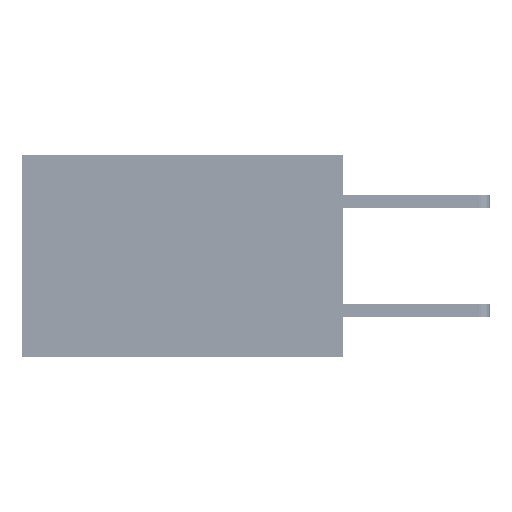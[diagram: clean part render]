
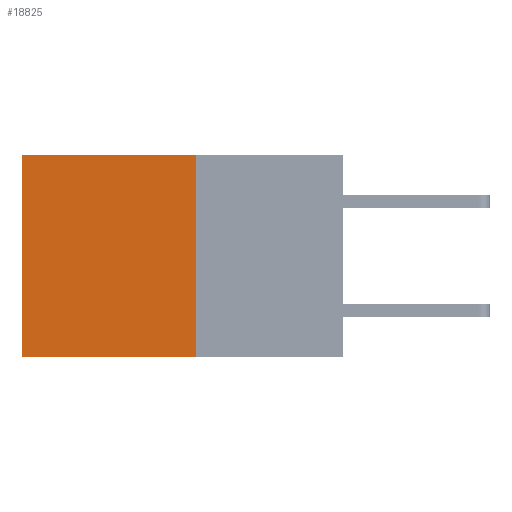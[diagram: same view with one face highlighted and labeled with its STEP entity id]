
A CAD part, left-side view. The second image highlights one B-rep face of the part: STEP entity #18825.
In plain terms, the highlighted planar face has unit normal (-1, 0, 0).
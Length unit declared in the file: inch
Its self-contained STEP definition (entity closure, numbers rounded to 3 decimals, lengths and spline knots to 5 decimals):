
#431 = FACE_OUTER_BOUND ( 'NONE', #22893, .T. ) ;
#1126 = CARTESIAN_POINT ( 'NONE',  ( 0.277, 0.27, 0. ) ) ;
#1893 = ORIENTED_EDGE ( 'NONE', *, *, #12973, .T. ) ;
#2403 = LINE ( 'NONE', #24866, #23224 ) ;
#3256 = CARTESIAN_POINT ( 'NONE',  ( 0.277, 0.59, 0. ) ) ;
#5105 = VERTEX_POINT ( 'NONE', #3256 ) ;
#5894 = DIRECTION ( 'NONE',  ( 1., 0., 0. ) ) ;
#6621 = CARTESIAN_POINT ( 'NONE',  ( 0.277, 0.27, -0.37 ) ) ;
#6742 = VECTOR ( 'NONE', #28355, 39.37008 ) ;
#7598 = ORIENTED_EDGE ( 'NONE', *, *, #15691, .T. ) ;
#7933 = VECTOR ( 'NONE', #16899, 39.37008 ) ;
#10224 = AXIS2_PLACEMENT_3D ( 'NONE', #14070, #5894, #19494 ) ;
#12973 = EDGE_CURVE ( 'NONE', #5105, #17827, #33513, .T. ) ;
#13945 = DIRECTION ( 'NONE',  ( 0., 0., -1. ) ) ;
#14070 = CARTESIAN_POINT ( 'NONE',  ( 0.277, 0.27, -0.37 ) ) ;
#14175 = CARTESIAN_POINT ( 'NONE',  ( 0.277, 0.27, 0. ) ) ;
#15649 = EDGE_CURVE ( 'NONE', #16264, #22211, #2403, .T. ) ;
#15691 = EDGE_CURVE ( 'NONE', #16264, #5105, #30457, .T. ) ;
#16264 = VERTEX_POINT ( 'NONE', #1126 ) ;
#16786 = PLANE ( 'NONE',  #10224 ) ;
#16899 = DIRECTION ( 'NONE',  ( 0., 1., 0. ) ) ;
#17827 = VERTEX_POINT ( 'NONE', #29131 ) ;
#18825 = ADVANCED_FACE ( 'NONE', ( #431 ), #16786, .F. ) ;
#19494 = DIRECTION ( 'NONE',  ( 0., 0., -1. ) ) ;
#22211 = VERTEX_POINT ( 'NONE', #25743 ) ;
#22426 = DIRECTION ( 'NONE',  ( 0., 0., -1. ) ) ;
#22840 = ORIENTED_EDGE ( 'NONE', *, *, #29817, .F. ) ;
#22893 = EDGE_LOOP ( 'NONE', ( #1893, #22840, #23657, #7598 ) ) ;
#23224 = VECTOR ( 'NONE', #13945, 39.37008 ) ;
#23657 = ORIENTED_EDGE ( 'NONE', *, *, #15649, .F. ) ;
#24866 = CARTESIAN_POINT ( 'NONE',  ( 0.277, 0.27, -0.37 ) ) ;
#25743 = CARTESIAN_POINT ( 'NONE',  ( 0.277, 0.27, -0.37 ) ) ;
#26260 = VECTOR ( 'NONE', #22426, 39.37008 ) ;
#28355 = DIRECTION ( 'NONE',  ( 0., 1., 0. ) ) ;
#28417 = LINE ( 'NONE', #6621, #6742 ) ;
#29131 = CARTESIAN_POINT ( 'NONE',  ( 0.277, 0.59, -0.37 ) ) ;
#29817 = EDGE_CURVE ( 'NONE', #22211, #17827, #28417, .T. ) ;
#30457 = LINE ( 'NONE', #14175, #7933 ) ;
#30504 = CARTESIAN_POINT ( 'NONE',  ( 0.277, 0.59, -0.37 ) ) ;
#33513 = LINE ( 'NONE', #30504, #26260 ) ;
